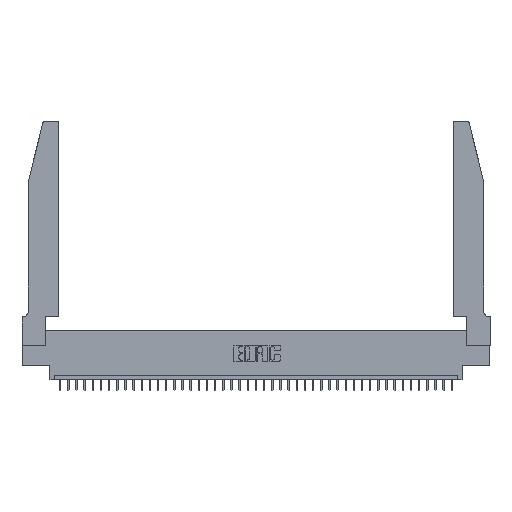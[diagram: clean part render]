
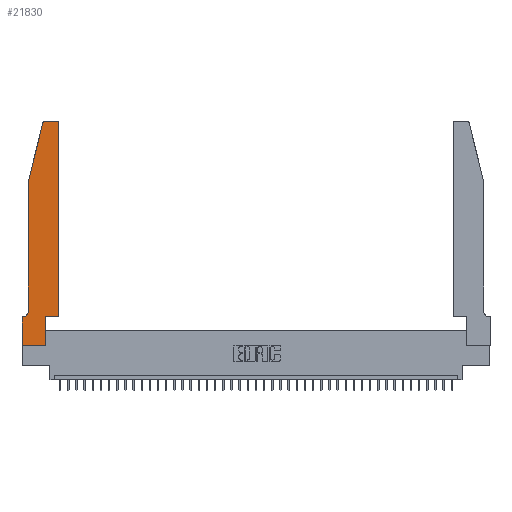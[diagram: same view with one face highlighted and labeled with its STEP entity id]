
A CAD part, top view. The second image highlights one B-rep face of the part: STEP entity #21830.
In plain terms, the highlighted planar face has unit normal (0, 0, 1).
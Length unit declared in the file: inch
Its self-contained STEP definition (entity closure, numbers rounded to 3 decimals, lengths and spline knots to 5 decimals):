
#402 = ORIENTED_EDGE ( 'NONE', *, *, #31294, .T. ) ;
#790 = VERTEX_POINT ( 'NONE', #34898 ) ;
#1004 = LINE ( 'NONE', #20001, #10766 ) ;
#1258 = EDGE_CURVE ( 'NONE', #32414, #22842, #11998, .T. ) ;
#2265 = CARTESIAN_POINT ( 'NONE',  ( 0.4505, 2.72, 0.37 ) ) ;
#3144 = CARTESIAN_POINT ( 'NONE',  ( 0.2865, 0.35, 0.37 ) ) ;
#3462 = EDGE_CURVE ( 'NONE', #40671, #790, #14799, .T. ) ;
#4849 = LINE ( 'NONE', #26566, #36757 ) ;
#5302 = AXIS2_PLACEMENT_3D ( 'NONE', #21952, #34611, #18024 ) ;
#5848 = DIRECTION ( 'NONE',  ( 1., 0., 0. ) ) ;
#6270 = CARTESIAN_POINT ( 'NONE',  ( 0.284, 2.72, 0.37 ) ) ;
#6394 = VERTEX_POINT ( 'NONE', #13739 ) ;
#6884 = AXIS2_PLACEMENT_3D ( 'NONE', #8183, #14573, #21405 ) ;
#6917 = VERTEX_POINT ( 'NONE', #20704 ) ;
#6999 = EDGE_CURVE ( 'NONE', #40325, #6917, #13210, .T. ) ;
#7912 = DIRECTION ( 'NONE',  ( 0., -1., 0. ) ) ;
#7977 = AXIS2_PLACEMENT_3D ( 'NONE', #6270, #19275, #5848 ) ;
#8183 = CARTESIAN_POINT ( 'NONE',  ( 0.4205, 2.72, 0.37 ) ) ;
#8329 = LINE ( 'NONE', #27161, #30026 ) ;
#9798 = VERTEX_POINT ( 'NONE', #30210 ) ;
#9932 = VECTOR ( 'NONE', #37358, 39.37008 ) ;
#10149 = VERTEX_POINT ( 'NONE', #18685 ) ;
#10716 = VERTEX_POINT ( 'NONE', #16904 ) ;
#10766 = VECTOR ( 'NONE', #29535, 39.37008 ) ;
#10808 = EDGE_CURVE ( 'NONE', #10716, #6394, #1004, .T. ) ;
#11533 = VECTOR ( 'NONE', #28553, 39.37008 ) ;
#11998 = LINE ( 'NONE', #12203, #26229 ) ;
#12203 = CARTESIAN_POINT ( 'NONE',  ( 0.2865, 0.35, 0.37 ) ) ;
#12311 = VERTEX_POINT ( 'NONE', #2265 ) ;
#12475 = EDGE_CURVE ( 'NONE', #22842, #30779, #15619, .T. ) ;
#12719 = CARTESIAN_POINT ( 'NONE',  ( 0.4505, 0.35, 0.37 ) ) ;
#13210 = CIRCLE ( 'NONE', #5302, 0.07 ) ;
#13635 = DIRECTION ( 'NONE',  ( 1., 0., 0. ) ) ;
#13739 = CARTESIAN_POINT ( 'NONE',  ( 0.0755, 2., 0.37 ) ) ;
#14250 = DIRECTION ( 'NONE',  ( 0., 0., 1. ) ) ;
#14573 = DIRECTION ( 'NONE',  ( 0., 0., 1. ) ) ;
#14744 = ORIENTED_EDGE ( 'NONE', *, *, #12475, .T. ) ;
#14799 = LINE ( 'NONE', #40067, #23677 ) ;
#15149 = LINE ( 'NONE', #39798, #9932 ) ;
#15619 = LINE ( 'NONE', #12719, #24659 ) ;
#15888 = DIRECTION ( 'NONE',  ( -1., 0., 0. ) ) ;
#16904 = CARTESIAN_POINT ( 'NONE',  ( 0.25487, 2.72718, 0.37 ) ) ;
#18024 = DIRECTION ( 'NONE',  ( -1., 0., 0. ) ) ;
#18685 = CARTESIAN_POINT ( 'NONE',  ( 0., 0., 0.37 ) ) ;
#19275 = DIRECTION ( 'NONE',  ( 0., 0., 1. ) ) ;
#20001 = CARTESIAN_POINT ( 'NONE',  ( 0.0755, 2., 0.37 ) ) ;
#20704 = CARTESIAN_POINT ( 'NONE',  ( 0.0055, 0.35, 0.37 ) ) ;
#21285 = CARTESIAN_POINT ( 'NONE',  ( 0.4505, 0.35, 0.37 ) ) ;
#21405 = DIRECTION ( 'NONE',  ( 1., 0., 0. ) ) ;
#21569 = ORIENTED_EDGE ( 'NONE', *, *, #3462, .T. ) ;
#21630 = CARTESIAN_POINT ( 'NONE',  ( 0.2865, 0., 0.37 ) ) ;
#21830 = ADVANCED_FACE ( 'NONE', ( #39342 ), #23590, .T. ) ;
#21901 = EDGE_CURVE ( 'NONE', #30779, #12311, #36879, .T. ) ;
#21932 = AXIS2_PLACEMENT_3D ( 'NONE', #32691, #14250, #13635 ) ;
#21952 = CARTESIAN_POINT ( 'NONE',  ( 0.0055, 0.42, 0.37 ) ) ;
#22517 = CIRCLE ( 'NONE', #7977, 0.03 ) ;
#22842 = VERTEX_POINT ( 'NONE', #3144 ) ;
#23590 = PLANE ( 'NONE',  #21932 ) ;
#23677 = VECTOR ( 'NONE', #15888, 39.37008 ) ;
#24659 = VECTOR ( 'NONE', #28063, 39.37008 ) ;
#24724 = CIRCLE ( 'NONE', #6884, 0.03 ) ;
#25455 = ORIENTED_EDGE ( 'NONE', *, *, #1258, .T. ) ;
#25645 = CARTESIAN_POINT ( 'NONE',  ( 0.0755, 2., 0.37 ) ) ;
#26078 = EDGE_CURVE ( 'NONE', #12311, #40671, #24724, .T. ) ;
#26229 = VECTOR ( 'NONE', #40778, 39.37008 ) ;
#26427 = EDGE_CURVE ( 'NONE', #9798, #10149, #8329, .T. ) ;
#26566 = CARTESIAN_POINT ( 'NONE',  ( 0., 0., 0.37 ) ) ;
#26590 = ORIENTED_EDGE ( 'NONE', *, *, #21901, .T. ) ;
#27161 = CARTESIAN_POINT ( 'NONE',  ( 0., 0., 0.37 ) ) ;
#27477 = CARTESIAN_POINT ( 'NONE',  ( 0.4505, 0.35, 0.37 ) ) ;
#27551 = EDGE_CURVE ( 'NONE', #10149, #32414, #4849, .T. ) ;
#27850 = LINE ( 'NONE', #25645, #11533 ) ;
#28063 = DIRECTION ( 'NONE',  ( 1., 0., 0. ) ) ;
#28553 = DIRECTION ( 'NONE',  ( 0., -1., 0. ) ) ;
#29419 = ORIENTED_EDGE ( 'NONE', *, *, #26427, .T. ) ;
#29535 = DIRECTION ( 'NONE',  ( -0.239, -0.971, 0. ) ) ;
#30026 = VECTOR ( 'NONE', #7912, 39.37008 ) ;
#30148 = ORIENTED_EDGE ( 'NONE', *, *, #31360, .T. ) ;
#30210 = CARTESIAN_POINT ( 'NONE',  ( 0., 0.35, 0.37 ) ) ;
#30779 = VERTEX_POINT ( 'NONE', #27477 ) ;
#31282 = ORIENTED_EDGE ( 'NONE', *, *, #6999, .T. ) ;
#31294 = EDGE_CURVE ( 'NONE', #6917, #9798, #15149, .T. ) ;
#31360 = EDGE_CURVE ( 'NONE', #790, #10716, #22517, .T. ) ;
#32414 = VERTEX_POINT ( 'NONE', #21630 ) ;
#32691 = CARTESIAN_POINT ( 'NONE',  ( 0., 0.35, 0.37 ) ) ;
#33121 = ORIENTED_EDGE ( 'NONE', *, *, #37429, .T. ) ;
#33414 = CARTESIAN_POINT ( 'NONE',  ( 0.0755, 0.42, 0.37 ) ) ;
#33506 = DIRECTION ( 'NONE',  ( 0., 1., 0. ) ) ;
#33749 = CARTESIAN_POINT ( 'NONE',  ( 0.4205, 2.75, 0.37 ) ) ;
#34611 = DIRECTION ( 'NONE',  ( 0., 0., -1. ) ) ;
#34700 = ORIENTED_EDGE ( 'NONE', *, *, #27551, .T. ) ;
#34852 = EDGE_LOOP ( 'NONE', ( #21569, #30148, #38023, #33121, #31282, #402, #29419, #34700, #25455, #14744, #26590, #37359 ) ) ;
#34898 = CARTESIAN_POINT ( 'NONE',  ( 0.284, 2.75, 0.37 ) ) ;
#36757 = VECTOR ( 'NONE', #38611, 39.37008 ) ;
#36879 = LINE ( 'NONE', #21285, #39152 ) ;
#37358 = DIRECTION ( 'NONE',  ( -1., 0., 0. ) ) ;
#37359 = ORIENTED_EDGE ( 'NONE', *, *, #26078, .T. ) ;
#37429 = EDGE_CURVE ( 'NONE', #6394, #40325, #27850, .T. ) ;
#38023 = ORIENTED_EDGE ( 'NONE', *, *, #10808, .T. ) ;
#38611 = DIRECTION ( 'NONE',  ( 1., 0., 0. ) ) ;
#39152 = VECTOR ( 'NONE', #33506, 39.37008 ) ;
#39342 = FACE_OUTER_BOUND ( 'NONE', #34852, .T. ) ;
#39798 = CARTESIAN_POINT ( 'NONE',  ( 0.0755, 0.35, 0.37 ) ) ;
#40067 = CARTESIAN_POINT ( 'NONE',  ( 0.2605, 2.75, 0.37 ) ) ;
#40325 = VERTEX_POINT ( 'NONE', #33414 ) ;
#40671 = VERTEX_POINT ( 'NONE', #33749 ) ;
#40778 = DIRECTION ( 'NONE',  ( 0., 1., 0. ) ) ;
